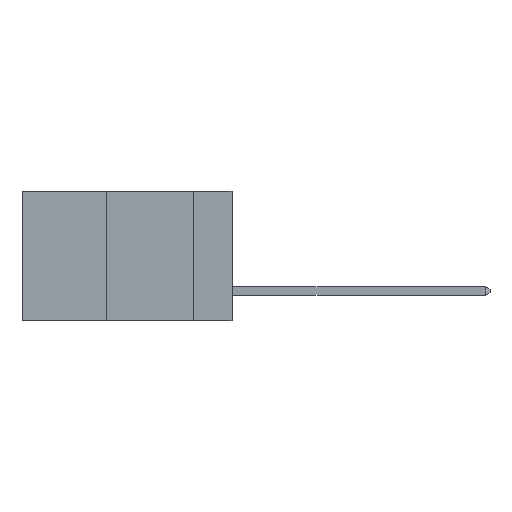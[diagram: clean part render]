
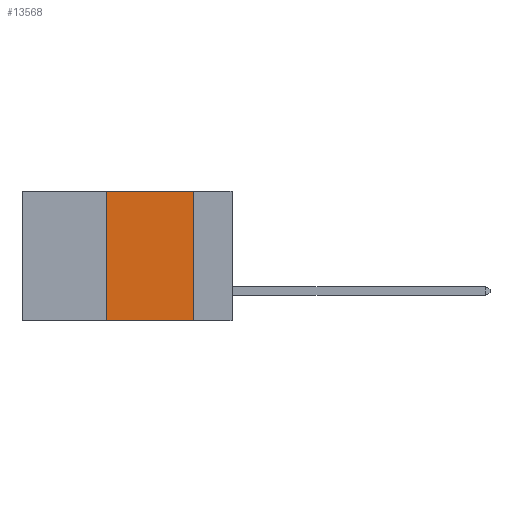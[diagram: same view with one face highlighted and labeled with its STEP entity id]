
A CAD part, left-side view. The second image highlights one B-rep face of the part: STEP entity #13568.
In plain terms, the highlighted planar face has unit normal (-1, 0, 0).
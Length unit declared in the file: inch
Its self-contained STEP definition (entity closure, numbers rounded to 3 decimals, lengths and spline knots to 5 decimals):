
#476 = DIRECTION ( 'NONE',  ( 0., -1., 0. ) ) ;
#1108 = VERTEX_POINT ( 'NONE', #11367 ) ;
#1208 = VECTOR ( 'NONE', #476, 39.37008 ) ;
#1493 = DIRECTION ( 'NONE',  ( 1., 0., 0. ) ) ;
#1933 = CARTESIAN_POINT ( 'NONE',  ( 0., 0.11, 0. ) ) ;
#2069 = CARTESIAN_POINT ( 'NONE',  ( 0., 0.36, -0.37 ) ) ;
#3494 = CARTESIAN_POINT ( 'NONE',  ( 0., 0.6, 0. ) ) ;
#3576 = ORIENTED_EDGE ( 'NONE', *, *, #3669, .F. ) ;
#3669 = EDGE_CURVE ( 'NONE', #15959, #1108, #6379, .T. ) ;
#3751 = EDGE_CURVE ( 'NONE', #15959, #4755, #11738, .T. ) ;
#4339 = CARTESIAN_POINT ( 'NONE',  ( 0., 0.6, -0.37 ) ) ;
#4755 = VERTEX_POINT ( 'NONE', #6041 ) ;
#5173 = VECTOR ( 'NONE', #8554, 39.37008 ) ;
#5423 = CARTESIAN_POINT ( 'NONE',  ( 0., 0.6, 0. ) ) ;
#6041 = CARTESIAN_POINT ( 'NONE',  ( 0., 0.11, -0.37 ) ) ;
#6379 = LINE ( 'NONE', #8151, #12930 ) ;
#8151 = CARTESIAN_POINT ( 'NONE',  ( 0., 0.36, 0. ) ) ;
#8554 = DIRECTION ( 'NONE',  ( 0., 0., -1. ) ) ;
#8965 = ORIENTED_EDGE ( 'NONE', *, *, #11875, .F. ) ;
#9492 = PLANE ( 'NONE',  #15218 ) ;
#9734 = DIRECTION ( 'NONE',  ( 0., 0., 1. ) ) ;
#9882 = EDGE_LOOP ( 'NONE', ( #8965, #11003, #3576, #12208 ) ) ;
#10785 = DIRECTION ( 'NONE',  ( 0., 0., -1. ) ) ;
#10993 = LINE ( 'NONE', #16241, #5173 ) ;
#11003 = ORIENTED_EDGE ( 'NONE', *, *, #13985, .F. ) ;
#11367 = CARTESIAN_POINT ( 'NONE',  ( 0., 0.36, 0. ) ) ;
#11738 = LINE ( 'NONE', #4339, #1208 ) ;
#11875 = EDGE_CURVE ( 'NONE', #16508, #4755, #10993, .T. ) ;
#12110 = FACE_OUTER_BOUND ( 'NONE', #9882, .T. ) ;
#12208 = ORIENTED_EDGE ( 'NONE', *, *, #3751, .T. ) ;
#12930 = VECTOR ( 'NONE', #9734, 39.37008 ) ;
#13277 = VECTOR ( 'NONE', #16502, 39.37008 ) ;
#13568 = ADVANCED_FACE ( 'NONE', ( #12110 ), #9492, .F. ) ;
#13985 = EDGE_CURVE ( 'NONE', #1108, #16508, #16622, .T. ) ;
#15218 = AXIS2_PLACEMENT_3D ( 'NONE', #5423, #1493, #10785 ) ;
#15959 = VERTEX_POINT ( 'NONE', #2069 ) ;
#16241 = CARTESIAN_POINT ( 'NONE',  ( 0., 0.11, 0. ) ) ;
#16502 = DIRECTION ( 'NONE',  ( 0., -1., 0. ) ) ;
#16508 = VERTEX_POINT ( 'NONE', #1933 ) ;
#16622 = LINE ( 'NONE', #3494, #13277 ) ;
